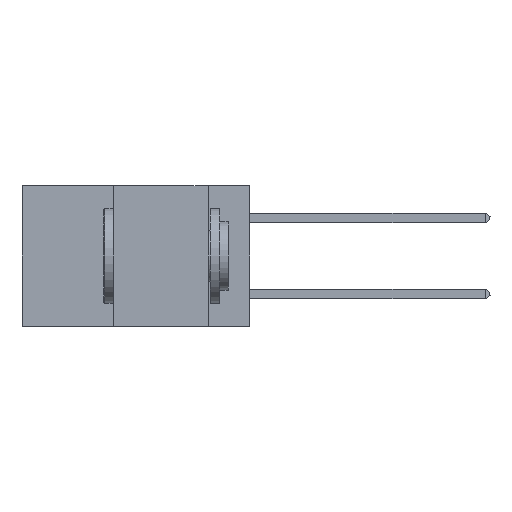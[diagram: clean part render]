
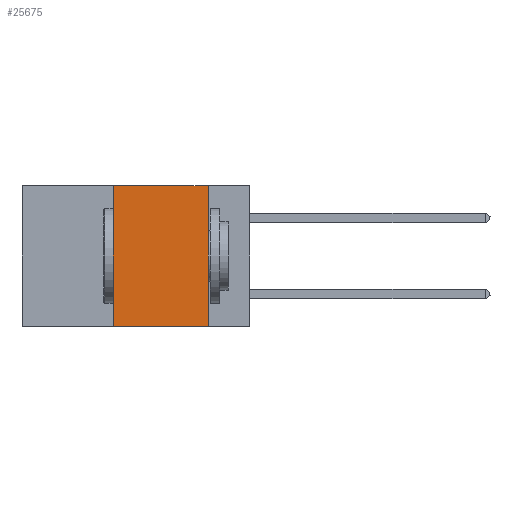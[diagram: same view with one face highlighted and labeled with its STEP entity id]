
A CAD part, left-side view. The second image highlights one B-rep face of the part: STEP entity #25675.
In plain terms, the highlighted planar face has unit normal (-1, 0, 0).
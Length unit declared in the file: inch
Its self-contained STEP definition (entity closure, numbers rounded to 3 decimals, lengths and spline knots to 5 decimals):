
#449 = AXIS2_PLACEMENT_3D ( 'NONE', #6952, #12881, #7340 ) ;
#2707 = ORIENTED_EDGE ( 'NONE', *, *, #16215, .T. ) ;
#3418 = LINE ( 'NONE', #34843, #35789 ) ;
#3588 = EDGE_CURVE ( 'NONE', #21830, #23416, #31168, .T. ) ;
#4444 = EDGE_CURVE ( 'NONE', #20561, #21830, #23244, .T. ) ;
#6633 = VECTOR ( 'NONE', #21743, 39.37008 ) ;
#6898 = EDGE_CURVE ( 'NONE', #32057, #20561, #3418, .T. ) ;
#6952 = CARTESIAN_POINT ( 'NONE',  ( 0., 0.6, 0. ) ) ;
#7340 = DIRECTION ( 'NONE',  ( 0., 0., -1. ) ) ;
#7611 = CARTESIAN_POINT ( 'NONE',  ( 0., 0.6, -0.37 ) ) ;
#8818 = DIRECTION ( 'NONE',  ( 0., -1., 0. ) ) ;
#10108 = ORIENTED_EDGE ( 'NONE', *, *, #6898, .F. ) ;
#10910 = ORIENTED_EDGE ( 'NONE', *, *, #3588, .F. ) ;
#11309 = DIRECTION ( 'NONE',  ( 0., 0., 1. ) ) ;
#12881 = DIRECTION ( 'NONE',  ( 1., 0., 0. ) ) ;
#16215 = EDGE_CURVE ( 'NONE', #32057, #23416, #21690, .T. ) ;
#16727 = VECTOR ( 'NONE', #8818, 39.37008 ) ;
#17376 = CARTESIAN_POINT ( 'NONE',  ( 0., 0.6, 0. ) ) ;
#17879 = CARTESIAN_POINT ( 'NONE',  ( 0., 0.36, -0.37 ) ) ;
#19412 = FACE_OUTER_BOUND ( 'NONE', #21017, .T. ) ;
#20561 = VERTEX_POINT ( 'NONE', #24423 ) ;
#21017 = EDGE_LOOP ( 'NONE', ( #10910, #36622, #10108, #2707 ) ) ;
#21690 = LINE ( 'NONE', #7611, #37873 ) ;
#21743 = DIRECTION ( 'NONE',  ( 0., 0., -1. ) ) ;
#21830 = VERTEX_POINT ( 'NONE', #38102 ) ;
#23244 = LINE ( 'NONE', #17376, #16727 ) ;
#23336 = CARTESIAN_POINT ( 'NONE',  ( 0., 0.11, -0.37 ) ) ;
#23416 = VERTEX_POINT ( 'NONE', #23336 ) ;
#24423 = CARTESIAN_POINT ( 'NONE',  ( 0., 0.36, 0. ) ) ;
#25675 = ADVANCED_FACE ( 'NONE', ( #19412 ), #31139, .F. ) ;
#28304 = DIRECTION ( 'NONE',  ( 0., -1., 0. ) ) ;
#31139 = PLANE ( 'NONE',  #449 ) ;
#31168 = LINE ( 'NONE', #33651, #6633 ) ;
#32057 = VERTEX_POINT ( 'NONE', #17879 ) ;
#33651 = CARTESIAN_POINT ( 'NONE',  ( 0., 0.11, 0. ) ) ;
#34843 = CARTESIAN_POINT ( 'NONE',  ( 0., 0.36, 0. ) ) ;
#35789 = VECTOR ( 'NONE', #11309, 39.37008 ) ;
#36622 = ORIENTED_EDGE ( 'NONE', *, *, #4444, .F. ) ;
#37873 = VECTOR ( 'NONE', #28304, 39.37008 ) ;
#38102 = CARTESIAN_POINT ( 'NONE',  ( 0., 0.11, 0. ) ) ;
